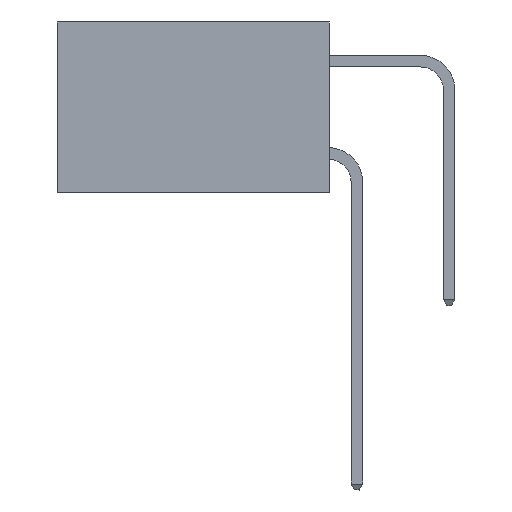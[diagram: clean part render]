
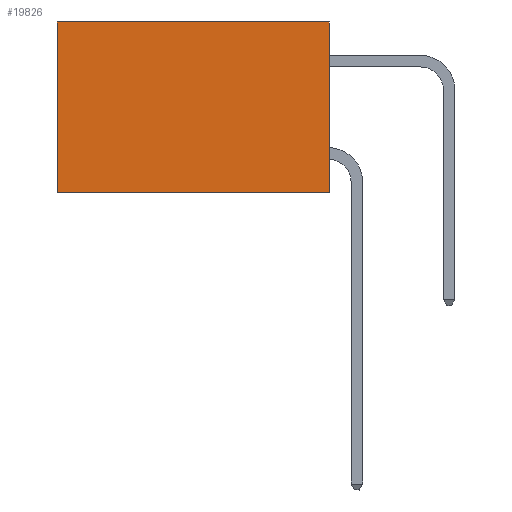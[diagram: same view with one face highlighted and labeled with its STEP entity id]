
A CAD part, left-side view. The second image highlights one B-rep face of the part: STEP entity #19826.
In plain terms, the highlighted planar face has unit normal (-1, 0, 0).
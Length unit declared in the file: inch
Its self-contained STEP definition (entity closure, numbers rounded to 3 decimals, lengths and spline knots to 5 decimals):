
#288 = ORIENTED_EDGE ( 'NONE', *, *, #1456, .F. ) ;
#1456 = EDGE_CURVE ( 'NONE', #15911, #27970, #18394, .T. ) ;
#3874 = DIRECTION ( 'NONE',  ( 0., 1., 0. ) ) ;
#4116 = VERTEX_POINT ( 'NONE', #23440 ) ;
#4443 = VECTOR ( 'NONE', #3874, 39.37008 ) ;
#4850 = EDGE_CURVE ( 'NONE', #17719, #4116, #16768, .T. ) ;
#7494 = DIRECTION ( 'NONE',  ( 1., 0., 0. ) ) ;
#7724 = CARTESIAN_POINT ( 'NONE',  ( 0.277, 0.59, 0. ) ) ;
#8814 = CARTESIAN_POINT ( 'NONE',  ( 0.277, 0., 0. ) ) ;
#10195 = ORIENTED_EDGE ( 'NONE', *, *, #21939, .T. ) ;
#11726 = DIRECTION ( 'NONE',  ( 0., 1., 0. ) ) ;
#12913 = EDGE_LOOP ( 'NONE', ( #15704, #20677, #288, #10195 ) ) ;
#13481 = AXIS2_PLACEMENT_3D ( 'NONE', #20607, #7494, #22783 ) ;
#14591 = CARTESIAN_POINT ( 'NONE',  ( 0.277, 0., -0.37 ) ) ;
#14788 = VECTOR ( 'NONE', #11726, 39.37008 ) ;
#15704 = ORIENTED_EDGE ( 'NONE', *, *, #4850, .T. ) ;
#15860 = PLANE ( 'NONE',  #13481 ) ;
#15911 = VERTEX_POINT ( 'NONE', #8814 ) ;
#16532 = CARTESIAN_POINT ( 'NONE',  ( 0.277, 0., -0.37 ) ) ;
#16768 = LINE ( 'NONE', #26951, #27609 ) ;
#17719 = VERTEX_POINT ( 'NONE', #7724 ) ;
#18394 = LINE ( 'NONE', #16532, #24827 ) ;
#19748 = FACE_OUTER_BOUND ( 'NONE', #12913, .T. ) ;
#19826 = ADVANCED_FACE ( 'NONE', ( #19748 ), #15860, .F. ) ;
#20607 = CARTESIAN_POINT ( 'NONE',  ( 0.277, 0., -0.37 ) ) ;
#20635 = LINE ( 'NONE', #14591, #4443 ) ;
#20677 = ORIENTED_EDGE ( 'NONE', *, *, #27900, .F. ) ;
#21939 = EDGE_CURVE ( 'NONE', #15911, #17719, #27809, .T. ) ;
#22510 = CARTESIAN_POINT ( 'NONE',  ( 0.277, 0., 0. ) ) ;
#22783 = DIRECTION ( 'NONE',  ( 0., 0., -1. ) ) ;
#23440 = CARTESIAN_POINT ( 'NONE',  ( 0.277, 0.59, -0.37 ) ) ;
#24827 = VECTOR ( 'NONE', #28321, 39.37008 ) ;
#26021 = CARTESIAN_POINT ( 'NONE',  ( 0.277, 0., -0.37 ) ) ;
#26767 = DIRECTION ( 'NONE',  ( 0., 0., -1. ) ) ;
#26951 = CARTESIAN_POINT ( 'NONE',  ( 0.277, 0.59, -0.37 ) ) ;
#27609 = VECTOR ( 'NONE', #26767, 39.37008 ) ;
#27809 = LINE ( 'NONE', #22510, #14788 ) ;
#27900 = EDGE_CURVE ( 'NONE', #27970, #4116, #20635, .T. ) ;
#27970 = VERTEX_POINT ( 'NONE', #26021 ) ;
#28321 = DIRECTION ( 'NONE',  ( 0., 0., -1. ) ) ;
